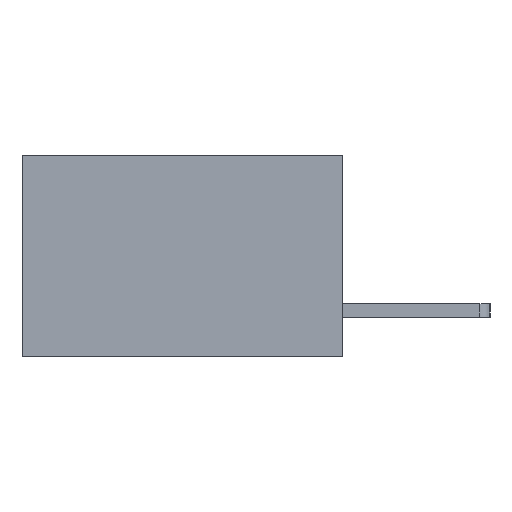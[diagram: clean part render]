
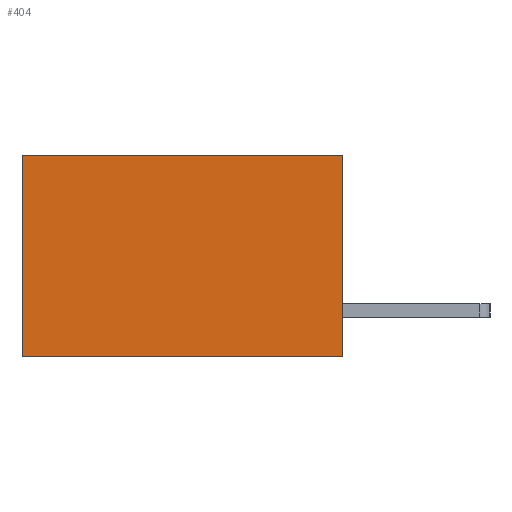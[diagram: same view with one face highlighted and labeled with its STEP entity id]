
A CAD part, left-side view. The second image highlights one B-rep face of the part: STEP entity #404.
In plain terms, the highlighted planar face has unit normal (-1, 0, 0).
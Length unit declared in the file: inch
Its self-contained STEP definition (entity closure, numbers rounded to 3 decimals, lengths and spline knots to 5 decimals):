
#82 = LINE ( 'NONE', #7382, #418 ) ;
#404 = ADVANCED_FACE ( 'NONE', ( #6344 ), #1537, .F. ) ;
#418 = VECTOR ( 'NONE', #1400, 39.37008 ) ;
#500 = VECTOR ( 'NONE', #8014, 39.37008 ) ;
#829 = LINE ( 'NONE', #7773, #500 ) ;
#1053 = DIRECTION ( 'NONE',  ( 1., 0., 0. ) ) ;
#1105 = EDGE_CURVE ( 'NONE', #4420, #1344, #9321, .T. ) ;
#1344 = VERTEX_POINT ( 'NONE', #7618 ) ;
#1351 = CARTESIAN_POINT ( 'NONE',  ( 0.277, 0., -0.37 ) ) ;
#1352 = ORIENTED_EDGE ( 'NONE', *, *, #5419, .T. ) ;
#1400 = DIRECTION ( 'NONE',  ( 0., 1., 0. ) ) ;
#1474 = ORIENTED_EDGE ( 'NONE', *, *, #10344, .F. ) ;
#1489 = DIRECTION ( 'NONE',  ( 0., 1., 0. ) ) ;
#1537 = PLANE ( 'NONE',  #4075 ) ;
#1563 = ORIENTED_EDGE ( 'NONE', *, *, #1105, .F. ) ;
#1573 = ORIENTED_EDGE ( 'NONE', *, *, #6581, .T. ) ;
#2306 = EDGE_LOOP ( 'NONE', ( #1352, #1474, #1563, #1573 ) ) ;
#4075 = AXIS2_PLACEMENT_3D ( 'NONE', #1351, #1053, #7842 ) ;
#4420 = VERTEX_POINT ( 'NONE', #10132 ) ;
#4443 = VECTOR ( 'NONE', #1489, 39.37008 ) ;
#4767 = LINE ( 'NONE', #6488, #4443 ) ;
#5419 = EDGE_CURVE ( 'NONE', #8731, #8539, #829, .T. ) ;
#6344 = FACE_OUTER_BOUND ( 'NONE', #2306, .T. ) ;
#6488 = CARTESIAN_POINT ( 'NONE',  ( 0.277, 0., 0. ) ) ;
#6581 = EDGE_CURVE ( 'NONE', #4420, #8731, #4767, .T. ) ;
#6876 = CARTESIAN_POINT ( 'NONE',  ( 0.277, 0.59, 0. ) ) ;
#7105 = VECTOR ( 'NONE', #9976, 39.37008 ) ;
#7382 = CARTESIAN_POINT ( 'NONE',  ( 0.277, 0., -0.37 ) ) ;
#7618 = CARTESIAN_POINT ( 'NONE',  ( 0.277, 0., -0.37 ) ) ;
#7715 = CARTESIAN_POINT ( 'NONE',  ( 0.277, 0.59, -0.37 ) ) ;
#7773 = CARTESIAN_POINT ( 'NONE',  ( 0.277, 0.59, -0.37 ) ) ;
#7842 = DIRECTION ( 'NONE',  ( 0., 0., -1. ) ) ;
#8014 = DIRECTION ( 'NONE',  ( 0., 0., -1. ) ) ;
#8539 = VERTEX_POINT ( 'NONE', #7715 ) ;
#8731 = VERTEX_POINT ( 'NONE', #6876 ) ;
#9321 = LINE ( 'NONE', #9578, #7105 ) ;
#9578 = CARTESIAN_POINT ( 'NONE',  ( 0.277, 0., -0.37 ) ) ;
#9976 = DIRECTION ( 'NONE',  ( 0., 0., -1. ) ) ;
#10132 = CARTESIAN_POINT ( 'NONE',  ( 0.277, 0., 0. ) ) ;
#10344 = EDGE_CURVE ( 'NONE', #1344, #8539, #82, .T. ) ;
